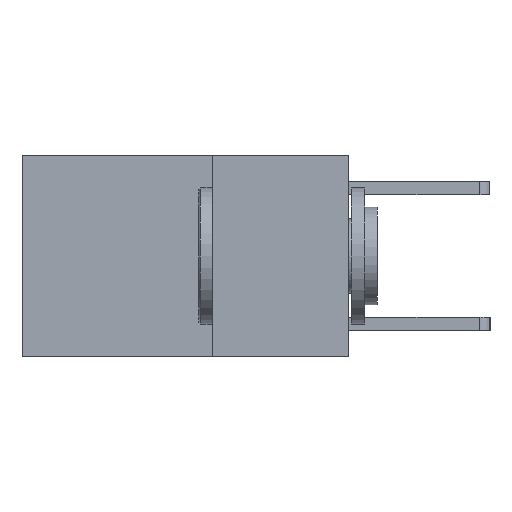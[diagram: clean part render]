
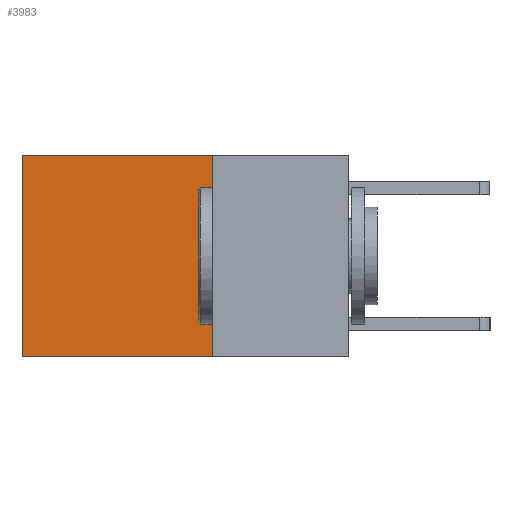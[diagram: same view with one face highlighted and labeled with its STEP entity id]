
A CAD part, left-side view. The second image highlights one B-rep face of the part: STEP entity #3983.
In plain terms, the highlighted planar face has unit normal (-1, 0, 0).
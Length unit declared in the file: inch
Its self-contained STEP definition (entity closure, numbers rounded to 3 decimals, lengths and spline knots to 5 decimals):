
#60 = VECTOR ( 'NONE', #1892, 39.37008 ) ;
#78 = ORIENTED_EDGE ( 'NONE', *, *, #6062, .F. ) ;
#232 = EDGE_CURVE ( 'NONE', #2927, #5585, #6406, .T. ) ;
#615 = VECTOR ( 'NONE', #7660, 39.37008 ) ;
#698 = VERTEX_POINT ( 'NONE', #756 ) ;
#730 = LINE ( 'NONE', #6946, #8090 ) ;
#756 = CARTESIAN_POINT ( 'NONE',  ( 0.2625, 0.25, -0.37 ) ) ;
#837 = DIRECTION ( 'NONE',  ( 0., 0., -1. ) ) ;
#849 = DIRECTION ( 'NONE',  ( 1., 0., 0. ) ) ;
#867 = PLANE ( 'NONE',  #3887 ) ;
#876 = CARTESIAN_POINT ( 'NONE',  ( 0.2625, 0.25, 0. ) ) ;
#1587 = CARTESIAN_POINT ( 'NONE',  ( 0.2625, 0.6, 0. ) ) ;
#1653 = EDGE_CURVE ( 'NONE', #6065, #698, #8198, .T. ) ;
#1892 = DIRECTION ( 'NONE',  ( 0., 1., 0. ) ) ;
#2746 = ORIENTED_EDGE ( 'NONE', *, *, #232, .T. ) ;
#2854 = VECTOR ( 'NONE', #6025, 39.37008 ) ;
#2927 = VERTEX_POINT ( 'NONE', #7486 ) ;
#3669 = ORIENTED_EDGE ( 'NONE', *, *, #7060, .T. ) ;
#3880 = LINE ( 'NONE', #7577, #60 ) ;
#3887 = AXIS2_PLACEMENT_3D ( 'NONE', #876, #849, #837 ) ;
#3983 = ADVANCED_FACE ( 'NONE', ( #4406 ), #867, .F. ) ;
#4144 = DIRECTION ( 'NONE',  ( 0., 1., 0. ) ) ;
#4406 = FACE_OUTER_BOUND ( 'NONE', #6917, .T. ) ;
#5585 = VERTEX_POINT ( 'NONE', #7100 ) ;
#6025 = DIRECTION ( 'NONE',  ( 0., 0., -1. ) ) ;
#6062 = EDGE_CURVE ( 'NONE', #698, #5585, #730, .T. ) ;
#6065 = VERTEX_POINT ( 'NONE', #8369 ) ;
#6406 = LINE ( 'NONE', #1587, #2854 ) ;
#6874 = ORIENTED_EDGE ( 'NONE', *, *, #1653, .F. ) ;
#6917 = EDGE_LOOP ( 'NONE', ( #2746, #78, #6874, #3669 ) ) ;
#6946 = CARTESIAN_POINT ( 'NONE',  ( 0.2625, 0.25, -0.37 ) ) ;
#7060 = EDGE_CURVE ( 'NONE', #6065, #2927, #3880, .T. ) ;
#7100 = CARTESIAN_POINT ( 'NONE',  ( 0.2625, 0.6, -0.37 ) ) ;
#7486 = CARTESIAN_POINT ( 'NONE',  ( 0.2625, 0.6, 0. ) ) ;
#7577 = CARTESIAN_POINT ( 'NONE',  ( 0.2625, 0.25, 0. ) ) ;
#7660 = DIRECTION ( 'NONE',  ( 0., 0., -1. ) ) ;
#7957 = CARTESIAN_POINT ( 'NONE',  ( 0.2625, 0.25, 0. ) ) ;
#8090 = VECTOR ( 'NONE', #4144, 39.37008 ) ;
#8198 = LINE ( 'NONE', #7957, #615 ) ;
#8369 = CARTESIAN_POINT ( 'NONE',  ( 0.2625, 0.25, 0. ) ) ;
